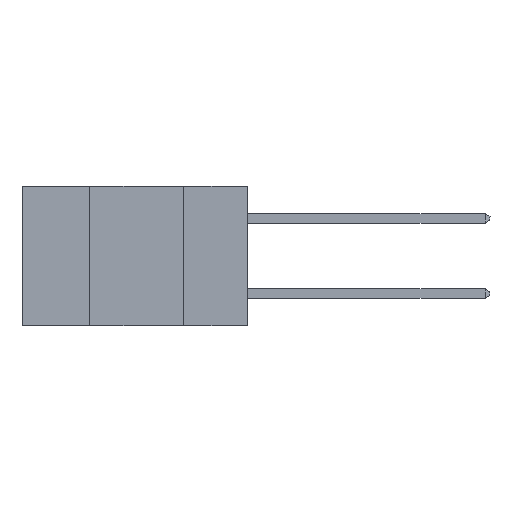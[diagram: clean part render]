
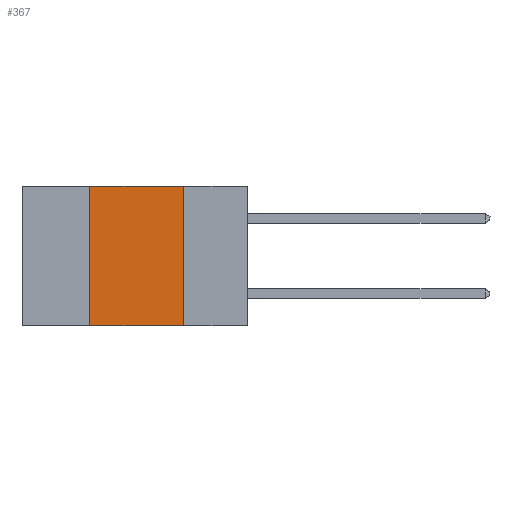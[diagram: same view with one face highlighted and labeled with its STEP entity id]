
A CAD part, left-side view. The second image highlights one B-rep face of the part: STEP entity #367.
In plain terms, the highlighted planar face has unit normal (-1, 0, 0).
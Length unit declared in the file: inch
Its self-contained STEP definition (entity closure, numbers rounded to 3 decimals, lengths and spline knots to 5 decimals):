
#69 = CARTESIAN_POINT ( 'NONE',  ( 0., 0.42, 0. ) ) ;
#367 = ADVANCED_FACE ( 'NONE', ( #669 ), #6527, .F. ) ;
#669 = FACE_OUTER_BOUND ( 'NONE', #6436, .T. ) ;
#780 = CARTESIAN_POINT ( 'NONE',  ( 0., 0.17, -0.37 ) ) ;
#1122 = DIRECTION ( 'NONE',  ( 0., -1., 0. ) ) ;
#1707 = ORIENTED_EDGE ( 'NONE', *, *, #4753, .F. ) ;
#1749 = ORIENTED_EDGE ( 'NONE', *, *, #2739, .F. ) ;
#1764 = VERTEX_POINT ( 'NONE', #5617 ) ;
#1904 = AXIS2_PLACEMENT_3D ( 'NONE', #4231, #2024, #8927 ) ;
#2024 = DIRECTION ( 'NONE',  ( 1., 0., 0. ) ) ;
#2294 = VERTEX_POINT ( 'NONE', #69 ) ;
#2380 = LINE ( 'NONE', #4623, #6958 ) ;
#2739 = EDGE_CURVE ( 'NONE', #2294, #1764, #3129, .T. ) ;
#2754 = EDGE_CURVE ( 'NONE', #8804, #3146, #6179, .T. ) ;
#3129 = LINE ( 'NONE', #7511, #4380 ) ;
#3146 = VERTEX_POINT ( 'NONE', #780 ) ;
#3776 = CARTESIAN_POINT ( 'NONE',  ( 0., 0.42, -0.37 ) ) ;
#3937 = ORIENTED_EDGE ( 'NONE', *, *, #7045, .F. ) ;
#4004 = CARTESIAN_POINT ( 'NONE',  ( 0., 0.6, -0.37 ) ) ;
#4231 = CARTESIAN_POINT ( 'NONE',  ( 0., 0.6, 0. ) ) ;
#4380 = VECTOR ( 'NONE', #6127, 39.37008 ) ;
#4389 = VECTOR ( 'NONE', #1122, 39.37008 ) ;
#4623 = CARTESIAN_POINT ( 'NONE',  ( 0., 0.17, -0.37 ) ) ;
#4739 = LINE ( 'NONE', #6268, #6880 ) ;
#4753 = EDGE_CURVE ( 'NONE', #1764, #3146, #2380, .T. ) ;
#5617 = CARTESIAN_POINT ( 'NONE',  ( 0., 0.17, 0. ) ) ;
#6127 = DIRECTION ( 'NONE',  ( 0., -1., 0. ) ) ;
#6150 = DIRECTION ( 'NONE',  ( 0., 0., -1. ) ) ;
#6179 = LINE ( 'NONE', #4004, #4389 ) ;
#6268 = CARTESIAN_POINT ( 'NONE',  ( 0., 0.42, -0.37 ) ) ;
#6436 = EDGE_LOOP ( 'NONE', ( #1707, #1749, #3937, #7129 ) ) ;
#6527 = PLANE ( 'NONE',  #1904 ) ;
#6880 = VECTOR ( 'NONE', #9209, 39.37008 ) ;
#6958 = VECTOR ( 'NONE', #6150, 39.37008 ) ;
#7045 = EDGE_CURVE ( 'NONE', #8804, #2294, #4739, .T. ) ;
#7129 = ORIENTED_EDGE ( 'NONE', *, *, #2754, .T. ) ;
#7511 = CARTESIAN_POINT ( 'NONE',  ( 0., 0.6, 0. ) ) ;
#8804 = VERTEX_POINT ( 'NONE', #3776 ) ;
#8927 = DIRECTION ( 'NONE',  ( 0., 0., -1. ) ) ;
#9209 = DIRECTION ( 'NONE',  ( 0., 0., 1. ) ) ;
